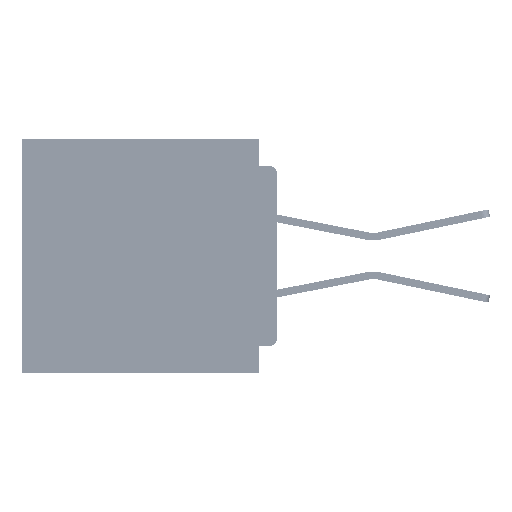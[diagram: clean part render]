
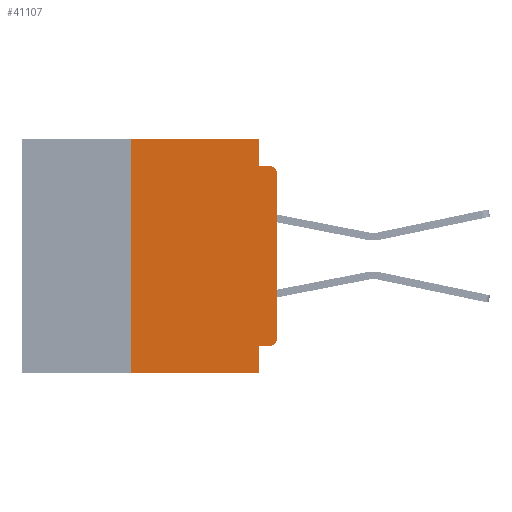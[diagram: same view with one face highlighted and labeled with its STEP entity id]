
A CAD part, left-side view. The second image highlights one B-rep face of the part: STEP entity #41107.
In plain terms, the highlighted planar face has unit normal (-1, 0, 0).
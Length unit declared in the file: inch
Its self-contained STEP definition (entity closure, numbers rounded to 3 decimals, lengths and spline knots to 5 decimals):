
#32 = LINE ( 'NONE', #50285, #40658 ) ;
#119 = VERTEX_POINT ( 'NONE', #3188 ) ;
#723 = CARTESIAN_POINT ( 'NONE',  ( 0., 0.437, -0.4 ) ) ;
#904 = DIRECTION ( 'NONE',  ( 0., 0., -1. ) ) ;
#2649 = DIRECTION ( 'NONE',  ( 0., 0., -1. ) ) ;
#3188 = CARTESIAN_POINT ( 'NONE',  ( 0., 0.25, 0. ) ) ;
#3404 = CARTESIAN_POINT ( 'NONE',  ( 0., 0.015, -0.045 ) ) ;
#3535 = VERTEX_POINT ( 'NONE', #46260 ) ;
#3923 = VERTEX_POINT ( 'NONE', #8068 ) ;
#6213 = EDGE_CURVE ( 'NONE', #3923, #31139, #32, .T. ) ;
#6282 = CARTESIAN_POINT ( 'NONE',  ( 0., 0.437, 0. ) ) ;
#6911 = DIRECTION ( 'NONE',  ( 0., 0., -1. ) ) ;
#7140 = EDGE_CURVE ( 'NONE', #32528, #50386, #51287, .T. ) ;
#8068 = CARTESIAN_POINT ( 'NONE',  ( 0., 0., -0.34 ) ) ;
#9663 = AXIS2_PLACEMENT_3D ( 'NONE', #18245, #55223, #23577 ) ;
#9760 = EDGE_CURVE ( 'NONE', #3535, #119, #31959, .T. ) ;
#10744 = VECTOR ( 'NONE', #66911, 39.37008 ) ;
#11755 = LINE ( 'NONE', #48319, #38206 ) ;
#11967 = VECTOR ( 'NONE', #2649, 39.37008 ) ;
#13488 = CIRCLE ( 'NONE', #9663, 0.015 ) ;
#14849 = AXIS2_PLACEMENT_3D ( 'NONE', #64299, #32641, #904 ) ;
#15529 = EDGE_CURVE ( 'NONE', #119, #40430, #41763, .T. ) ;
#16540 = DIRECTION ( 'NONE',  ( 0., -1., 0. ) ) ;
#17377 = PLANE ( 'NONE',  #17401 ) ;
#17401 = AXIS2_PLACEMENT_3D ( 'NONE', #59672, #38618, #6911 ) ;
#17988 = ORIENTED_EDGE ( 'NONE', *, *, #7140, .F. ) ;
#18016 = EDGE_CURVE ( 'NONE', #65762, #19642, #11755, .T. ) ;
#18245 = CARTESIAN_POINT ( 'NONE',  ( 0., 0.015, -0.34 ) ) ;
#18633 = DIRECTION ( 'NONE',  ( 0., 0., 1. ) ) ;
#19502 = CARTESIAN_POINT ( 'NONE',  ( 0., 0.25, -0.4 ) ) ;
#19642 = VERTEX_POINT ( 'NONE', #3404 ) ;
#22822 = CARTESIAN_POINT ( 'NONE',  ( 0., 0.031, 0. ) ) ;
#23577 = DIRECTION ( 'NONE',  ( 0., 0., -1. ) ) ;
#24043 = EDGE_CURVE ( 'NONE', #31139, #19642, #47231, .T. ) ;
#26085 = LINE ( 'NONE', #723, #52510 ) ;
#27253 = FACE_OUTER_BOUND ( 'NONE', #46428, .T. ) ;
#27746 = ORIENTED_EDGE ( 'NONE', *, *, #24043, .T. ) ;
#28842 = EDGE_CURVE ( 'NONE', #3535, #41755, #26085, .T. ) ;
#30110 = DIRECTION ( 'NONE',  ( 0., 0., 1. ) ) ;
#30321 = VECTOR ( 'NONE', #30110, 39.37008 ) ;
#31139 = VERTEX_POINT ( 'NONE', #48285 ) ;
#31631 = CARTESIAN_POINT ( 'NONE',  ( 0., 0., -0.355 ) ) ;
#31959 = LINE ( 'NONE', #19502, #30321 ) ;
#32334 = EDGE_CURVE ( 'NONE', #50386, #41755, #63529, .T. ) ;
#32528 = VERTEX_POINT ( 'NONE', #54284 ) ;
#32641 = DIRECTION ( 'NONE',  ( -1., 0., 0. ) ) ;
#33952 = CARTESIAN_POINT ( 'NONE',  ( 0., 0.031, -0.355 ) ) ;
#34361 = CARTESIAN_POINT ( 'NONE',  ( 0., 0.031, 0. ) ) ;
#38127 = EDGE_CURVE ( 'NONE', #40430, #65762, #38418, .T. ) ;
#38162 = ORIENTED_EDGE ( 'NONE', *, *, #63855, .T. ) ;
#38206 = VECTOR ( 'NONE', #53616, 39.37008 ) ;
#38418 = LINE ( 'NONE', #34361, #11967 ) ;
#38618 = DIRECTION ( 'NONE',  ( 1., 0., 0. ) ) ;
#40430 = VERTEX_POINT ( 'NONE', #22822 ) ;
#40658 = VECTOR ( 'NONE', #18633, 39.37008 ) ;
#41012 = ORIENTED_EDGE ( 'NONE', *, *, #15529, .F. ) ;
#41107 = ADVANCED_FACE ( 'NONE', ( #27253 ), #17377, .F. ) ;
#41755 = VERTEX_POINT ( 'NONE', #43409 ) ;
#41763 = LINE ( 'NONE', #6282, #55869 ) ;
#43409 = CARTESIAN_POINT ( 'NONE',  ( 0., 0.031, -0.4 ) ) ;
#43418 = ORIENTED_EDGE ( 'NONE', *, *, #28842, .T. ) ;
#46260 = CARTESIAN_POINT ( 'NONE',  ( 0., 0.25, -0.4 ) ) ;
#46428 = EDGE_LOOP ( 'NONE', ( #59010, #27746, #49239, #67500, #41012, #61592, #43418, #63622, #17988, #38162 ) ) ;
#47231 = CIRCLE ( 'NONE', #14849, 0.015 ) ;
#47344 = CARTESIAN_POINT ( 'NONE',  ( 0., 0.031, -0.4 ) ) ;
#48285 = CARTESIAN_POINT ( 'NONE',  ( 0., 0., -0.06 ) ) ;
#48319 = CARTESIAN_POINT ( 'NONE',  ( 0., 0., -0.045 ) ) ;
#48625 = DIRECTION ( 'NONE',  ( 0., -1., 0. ) ) ;
#49239 = ORIENTED_EDGE ( 'NONE', *, *, #18016, .F. ) ;
#49483 = VECTOR ( 'NONE', #57993, 39.37008 ) ;
#50285 = CARTESIAN_POINT ( 'NONE',  ( 0., 0., 0. ) ) ;
#50386 = VERTEX_POINT ( 'NONE', #33952 ) ;
#51287 = LINE ( 'NONE', #31631, #10744 ) ;
#52510 = VECTOR ( 'NONE', #16540, 39.37008 ) ;
#53616 = DIRECTION ( 'NONE',  ( 0., -1., 0. ) ) ;
#54284 = CARTESIAN_POINT ( 'NONE',  ( 0., 0.015, -0.355 ) ) ;
#55223 = DIRECTION ( 'NONE',  ( -1., 0., 0. ) ) ;
#55869 = VECTOR ( 'NONE', #48625, 39.37008 ) ;
#57993 = DIRECTION ( 'NONE',  ( 0., 0., -1. ) ) ;
#59010 = ORIENTED_EDGE ( 'NONE', *, *, #6213, .T. ) ;
#59672 = CARTESIAN_POINT ( 'NONE',  ( 0., 0.437, 0. ) ) ;
#61592 = ORIENTED_EDGE ( 'NONE', *, *, #9760, .F. ) ;
#63529 = LINE ( 'NONE', #47344, #49483 ) ;
#63622 = ORIENTED_EDGE ( 'NONE', *, *, #32334, .F. ) ;
#63855 = EDGE_CURVE ( 'NONE', #32528, #3923, #13488, .T. ) ;
#64299 = CARTESIAN_POINT ( 'NONE',  ( 0., 0.015, -0.06 ) ) ;
#65762 = VERTEX_POINT ( 'NONE', #66725 ) ;
#66725 = CARTESIAN_POINT ( 'NONE',  ( 0., 0.031, -0.045 ) ) ;
#66911 = DIRECTION ( 'NONE',  ( 0., 1., 0. ) ) ;
#67500 = ORIENTED_EDGE ( 'NONE', *, *, #38127, .F. ) ;
